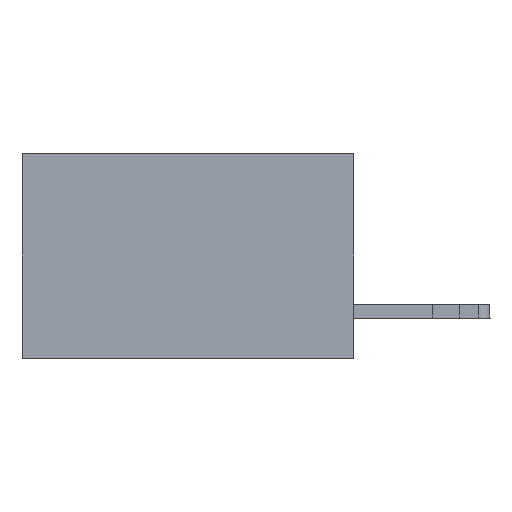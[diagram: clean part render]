
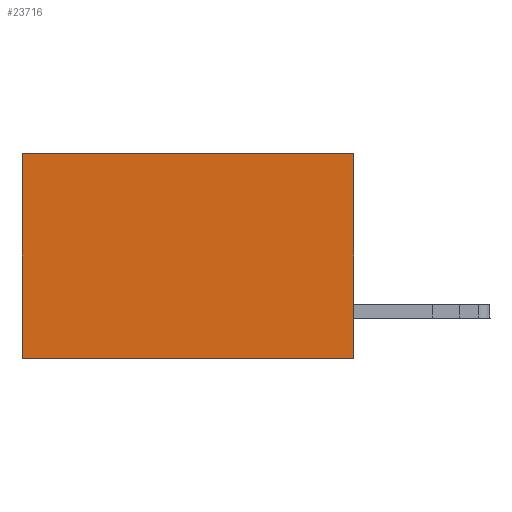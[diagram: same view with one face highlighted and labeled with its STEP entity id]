
A CAD part, left-side view. The second image highlights one B-rep face of the part: STEP entity #23716.
In plain terms, the highlighted planar face has unit normal (-1, 0, 0).
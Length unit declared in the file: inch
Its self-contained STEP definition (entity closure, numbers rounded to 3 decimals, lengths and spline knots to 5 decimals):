
#1368 = DIRECTION ( 'NONE',  ( 0., 1., 0. ) ) ;
#2618 = LINE ( 'NONE', #26002, #24345 ) ;
#2960 = AXIS2_PLACEMENT_3D ( 'NONE', #29333, #14716, #35107 ) ;
#3645 = CARTESIAN_POINT ( 'NONE',  ( 0.2875, 0., 0. ) ) ;
#3714 = EDGE_LOOP ( 'NONE', ( #22482, #34535, #37679, #14124 ) ) ;
#6918 = LINE ( 'NONE', #7451, #14741 ) ;
#7451 = CARTESIAN_POINT ( 'NONE',  ( 0.2875, 0., 0. ) ) ;
#9796 = CARTESIAN_POINT ( 'NONE',  ( 0.2875, 0.6, 0. ) ) ;
#10409 = CARTESIAN_POINT ( 'NONE',  ( 0.2875, 0., -0.37 ) ) ;
#11015 = VECTOR ( 'NONE', #26649, 39.37008 ) ;
#13367 = DIRECTION ( 'NONE',  ( 0., 0., -1. ) ) ;
#14124 = ORIENTED_EDGE ( 'NONE', *, *, #20979, .T. ) ;
#14716 = DIRECTION ( 'NONE',  ( 1., 0., 0. ) ) ;
#14741 = VECTOR ( 'NONE', #13367, 39.37008 ) ;
#14969 = CARTESIAN_POINT ( 'NONE',  ( 0.2875, 0., -0.37 ) ) ;
#15020 = CARTESIAN_POINT ( 'NONE',  ( 0.2875, 0.6, -0.37 ) ) ;
#19073 = VERTEX_POINT ( 'NONE', #14969 ) ;
#19793 = VERTEX_POINT ( 'NONE', #3645 ) ;
#19973 = EDGE_CURVE ( 'NONE', #19793, #19073, #6918, .T. ) ;
#20801 = EDGE_CURVE ( 'NONE', #33958, #26859, #2618, .T. ) ;
#20979 = EDGE_CURVE ( 'NONE', #19793, #33958, #28427, .T. ) ;
#22022 = LINE ( 'NONE', #10409, #30683 ) ;
#22482 = ORIENTED_EDGE ( 'NONE', *, *, #20801, .T. ) ;
#23067 = DIRECTION ( 'NONE',  ( 0., 0., -1. ) ) ;
#23481 = PLANE ( 'NONE',  #2960 ) ;
#23716 = ADVANCED_FACE ( 'NONE', ( #34759 ), #23481, .F. ) ;
#24345 = VECTOR ( 'NONE', #23067, 39.37008 ) ;
#25197 = EDGE_CURVE ( 'NONE', #19073, #26859, #22022, .T. ) ;
#26002 = CARTESIAN_POINT ( 'NONE',  ( 0.2875, 0.6, 0. ) ) ;
#26649 = DIRECTION ( 'NONE',  ( 0., 1., 0. ) ) ;
#26859 = VERTEX_POINT ( 'NONE', #15020 ) ;
#28427 = LINE ( 'NONE', #35342, #11015 ) ;
#29333 = CARTESIAN_POINT ( 'NONE',  ( 0.2875, 0., 0. ) ) ;
#30683 = VECTOR ( 'NONE', #1368, 39.37008 ) ;
#33958 = VERTEX_POINT ( 'NONE', #9796 ) ;
#34535 = ORIENTED_EDGE ( 'NONE', *, *, #25197, .F. ) ;
#34759 = FACE_OUTER_BOUND ( 'NONE', #3714, .T. ) ;
#35107 = DIRECTION ( 'NONE',  ( 0., 0., -1. ) ) ;
#35342 = CARTESIAN_POINT ( 'NONE',  ( 0.2875, 0., 0. ) ) ;
#37679 = ORIENTED_EDGE ( 'NONE', *, *, #19973, .F. ) ;
